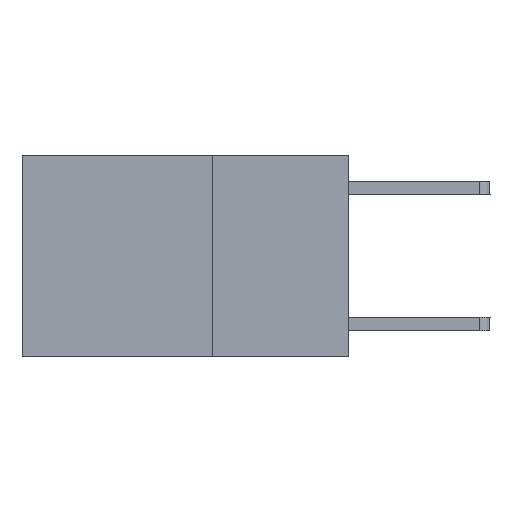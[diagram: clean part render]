
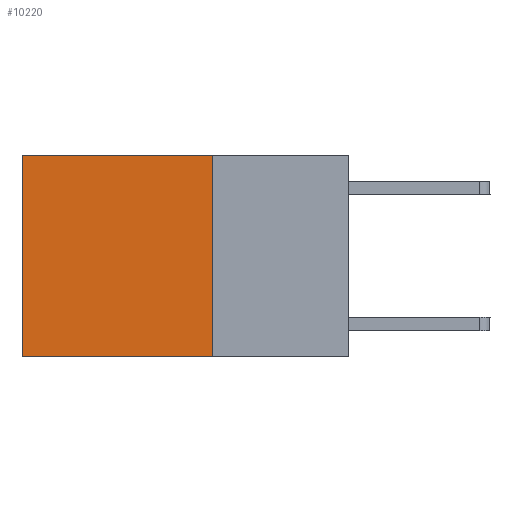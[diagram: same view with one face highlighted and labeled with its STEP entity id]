
A CAD part, left-side view. The second image highlights one B-rep face of the part: STEP entity #10220.
In plain terms, the highlighted planar face has unit normal (-1, 0, 0).
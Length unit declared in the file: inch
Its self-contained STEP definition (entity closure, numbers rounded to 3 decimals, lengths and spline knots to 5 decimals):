
#40 = VERTEX_POINT ( 'NONE', #5588 ) ;
#1414 = CARTESIAN_POINT ( 'NONE',  ( 0.2625, 0.25, 0. ) ) ;
#1459 = LINE ( 'NONE', #6319, #4239 ) ;
#1909 = CARTESIAN_POINT ( 'NONE',  ( 0.2625, 0.25, -0.37 ) ) ;
#2337 = ORIENTED_EDGE ( 'NONE', *, *, #4537, .F. ) ;
#2360 = ORIENTED_EDGE ( 'NONE', *, *, #7749, .T. ) ;
#2565 = ORIENTED_EDGE ( 'NONE', *, *, #10026, .T. ) ;
#2664 = CARTESIAN_POINT ( 'NONE',  ( 0.2625, 0.6, 0. ) ) ;
#2819 = VECTOR ( 'NONE', #6897, 39.37008 ) ;
#2838 = CARTESIAN_POINT ( 'NONE',  ( 0.2625, 0.25, 0. ) ) ;
#3067 = FACE_OUTER_BOUND ( 'NONE', #8794, .T. ) ;
#3373 = VERTEX_POINT ( 'NONE', #1909 ) ;
#3430 = EDGE_CURVE ( 'NONE', #3373, #8127, #1459, .T. ) ;
#3451 = LINE ( 'NONE', #6751, #6723 ) ;
#4239 = VECTOR ( 'NONE', #10563, 39.37008 ) ;
#4537 = EDGE_CURVE ( 'NONE', #40, #3373, #3451, .T. ) ;
#5217 = AXIS2_PLACEMENT_3D ( 'NONE', #1414, #9707, #8074 ) ;
#5415 = VERTEX_POINT ( 'NONE', #2664 ) ;
#5588 = CARTESIAN_POINT ( 'NONE',  ( 0.2625, 0.25, 0. ) ) ;
#6014 = LINE ( 'NONE', #10310, #7468 ) ;
#6319 = CARTESIAN_POINT ( 'NONE',  ( 0.2625, 0.25, -0.37 ) ) ;
#6723 = VECTOR ( 'NONE', #6793, 39.37008 ) ;
#6751 = CARTESIAN_POINT ( 'NONE',  ( 0.2625, 0.25, 0. ) ) ;
#6793 = DIRECTION ( 'NONE',  ( 0., 0., -1. ) ) ;
#6897 = DIRECTION ( 'NONE',  ( 0., 1., 0. ) ) ;
#6901 = DIRECTION ( 'NONE',  ( 0., 0., -1. ) ) ;
#7468 = VECTOR ( 'NONE', #6901, 39.37008 ) ;
#7749 = EDGE_CURVE ( 'NONE', #40, #5415, #10369, .T. ) ;
#7826 = CARTESIAN_POINT ( 'NONE',  ( 0.2625, 0.6, -0.37 ) ) ;
#8074 = DIRECTION ( 'NONE',  ( 0., 0., -1. ) ) ;
#8127 = VERTEX_POINT ( 'NONE', #7826 ) ;
#8794 = EDGE_LOOP ( 'NONE', ( #2565, #10736, #2337, #2360 ) ) ;
#8851 = PLANE ( 'NONE',  #5217 ) ;
#9707 = DIRECTION ( 'NONE',  ( 1., 0., 0. ) ) ;
#10026 = EDGE_CURVE ( 'NONE', #5415, #8127, #6014, .T. ) ;
#10220 = ADVANCED_FACE ( 'NONE', ( #3067 ), #8851, .F. ) ;
#10310 = CARTESIAN_POINT ( 'NONE',  ( 0.2625, 0.6, 0. ) ) ;
#10369 = LINE ( 'NONE', #2838, #2819 ) ;
#10563 = DIRECTION ( 'NONE',  ( 0., 1., 0. ) ) ;
#10736 = ORIENTED_EDGE ( 'NONE', *, *, #3430, .F. ) ;
